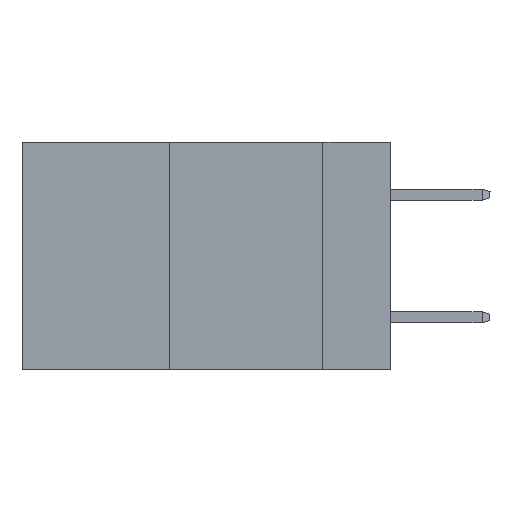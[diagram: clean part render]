
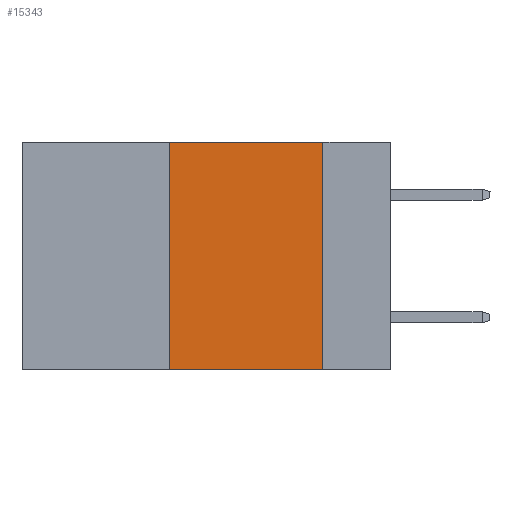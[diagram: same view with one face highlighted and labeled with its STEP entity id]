
A CAD part, left-side view. The second image highlights one B-rep face of the part: STEP entity #15343.
In plain terms, the highlighted planar face has unit normal (-1, 0, 0).
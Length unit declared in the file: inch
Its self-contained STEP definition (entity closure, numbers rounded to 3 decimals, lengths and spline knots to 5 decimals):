
#734 = VERTEX_POINT ( 'NONE', #16669 ) ;
#1079 = LINE ( 'NONE', #20890, #7413 ) ;
#1442 = VERTEX_POINT ( 'NONE', #8744 ) ;
#2525 = CARTESIAN_POINT ( 'NONE',  ( 0., 0.11, 0. ) ) ;
#2993 = EDGE_CURVE ( 'NONE', #9865, #734, #20574, .T. ) ;
#5864 = VECTOR ( 'NONE', #15488, 39.37008 ) ;
#6515 = DIRECTION ( 'NONE',  ( 1., 0., 0. ) ) ;
#6728 = ORIENTED_EDGE ( 'NONE', *, *, #18005, .F. ) ;
#7174 = VERTEX_POINT ( 'NONE', #9802 ) ;
#7413 = VECTOR ( 'NONE', #12127, 39.37008 ) ;
#7833 = FACE_OUTER_BOUND ( 'NONE', #10923, .T. ) ;
#8583 = EDGE_CURVE ( 'NONE', #1442, #9865, #1079, .T. ) ;
#8744 = CARTESIAN_POINT ( 'NONE',  ( 0., 0.36, 0. ) ) ;
#9595 = ORIENTED_EDGE ( 'NONE', *, *, #17537, .T. ) ;
#9723 = LINE ( 'NONE', #17542, #12175 ) ;
#9802 = CARTESIAN_POINT ( 'NONE',  ( 0., 0.36, -0.37 ) ) ;
#9865 = VERTEX_POINT ( 'NONE', #19032 ) ;
#10923 = EDGE_LOOP ( 'NONE', ( #21753, #11504, #6728, #9595 ) ) ;
#11504 = ORIENTED_EDGE ( 'NONE', *, *, #8583, .F. ) ;
#12127 = DIRECTION ( 'NONE',  ( 0., -1., 0. ) ) ;
#12175 = VECTOR ( 'NONE', #12201, 39.37008 ) ;
#12201 = DIRECTION ( 'NONE',  ( 0., -1., 0. ) ) ;
#13040 = DIRECTION ( 'NONE',  ( 0., 0., -1. ) ) ;
#13581 = DIRECTION ( 'NONE',  ( 0., 0., -1. ) ) ;
#15197 = LINE ( 'NONE', #22481, #5864 ) ;
#15343 = ADVANCED_FACE ( 'NONE', ( #7833 ), #22497, .F. ) ;
#15488 = DIRECTION ( 'NONE',  ( 0., 0., 1. ) ) ;
#15508 = CARTESIAN_POINT ( 'NONE',  ( 0., 0.6, 0. ) ) ;
#16318 = AXIS2_PLACEMENT_3D ( 'NONE', #15508, #6515, #13581 ) ;
#16669 = CARTESIAN_POINT ( 'NONE',  ( 0., 0.11, -0.37 ) ) ;
#17537 = EDGE_CURVE ( 'NONE', #7174, #734, #9723, .T. ) ;
#17542 = CARTESIAN_POINT ( 'NONE',  ( 0., 0.6, -0.37 ) ) ;
#18005 = EDGE_CURVE ( 'NONE', #7174, #1442, #15197, .T. ) ;
#18396 = VECTOR ( 'NONE', #13040, 39.37008 ) ;
#19032 = CARTESIAN_POINT ( 'NONE',  ( 0., 0.11, 0. ) ) ;
#20574 = LINE ( 'NONE', #2525, #18396 ) ;
#20890 = CARTESIAN_POINT ( 'NONE',  ( 0., 0.6, 0. ) ) ;
#21753 = ORIENTED_EDGE ( 'NONE', *, *, #2993, .F. ) ;
#22481 = CARTESIAN_POINT ( 'NONE',  ( 0., 0.36, 0. ) ) ;
#22497 = PLANE ( 'NONE',  #16318 ) ;
